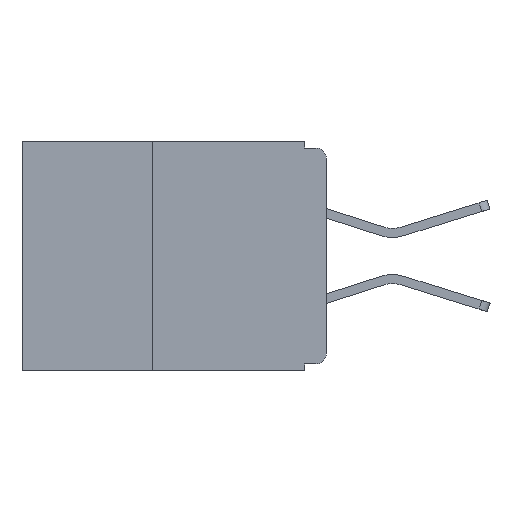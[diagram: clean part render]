
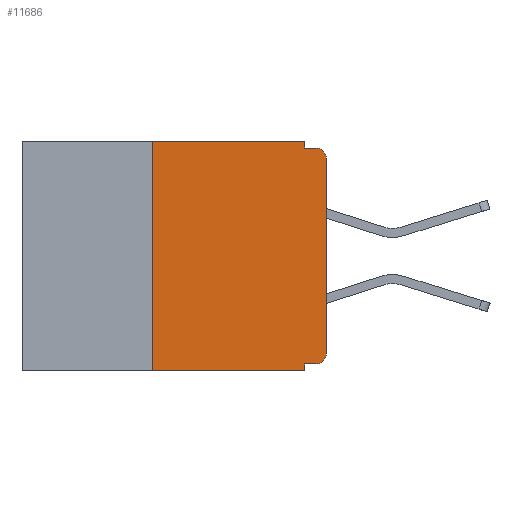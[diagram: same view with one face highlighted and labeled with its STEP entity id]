
A CAD part, left-side view. The second image highlights one B-rep face of the part: STEP entity #11686.
In plain terms, the highlighted planar face has unit normal (-1, 0, 0).
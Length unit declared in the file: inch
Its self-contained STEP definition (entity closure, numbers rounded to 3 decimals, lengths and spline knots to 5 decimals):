
#15 = AXIS2_PLACEMENT_3D ( 'NONE', #8913, #19501, #10410 ) ;
#579 = CARTESIAN_POINT ( 'NONE',  ( 0., 0.015, -0.025 ) ) ;
#1544 = CARTESIAN_POINT ( 'NONE',  ( 0., 0.437, -0.33 ) ) ;
#1584 = LINE ( 'NONE', #1544, #12838 ) ;
#1586 = DIRECTION ( 'NONE',  ( 0., 1., 0. ) ) ;
#1719 = AXIS2_PLACEMENT_3D ( 'NONE', #579, #11249, #2128 ) ;
#2058 = DIRECTION ( 'NONE',  ( 0., -1., 0. ) ) ;
#2121 = CARTESIAN_POINT ( 'NONE',  ( 0., 0., -0.025 ) ) ;
#2128 = DIRECTION ( 'NONE',  ( 0., 0., -1. ) ) ;
#2488 = FACE_OUTER_BOUND ( 'NONE', #13505, .T. ) ;
#2527 = VECTOR ( 'NONE', #3831, 39.37008 ) ;
#3099 = ORIENTED_EDGE ( 'NONE', *, *, #18047, .F. ) ;
#3177 = DIRECTION ( 'NONE',  ( 1., 0., 0. ) ) ;
#3681 = EDGE_CURVE ( 'NONE', #10361, #7495, #19598, .T. ) ;
#3831 = DIRECTION ( 'NONE',  ( 0., 0., -1. ) ) ;
#3846 = CARTESIAN_POINT ( 'NONE',  ( 0., 0.031, -0.33 ) ) ;
#4240 = LINE ( 'NONE', #17031, #7351 ) ;
#4249 = VERTEX_POINT ( 'NONE', #2121 ) ;
#4680 = VERTEX_POINT ( 'NONE', #13640 ) ;
#4694 = CARTESIAN_POINT ( 'NONE',  ( 0., 0., -0.32 ) ) ;
#5428 = EDGE_CURVE ( 'NONE', #9718, #18301, #8872, .T. ) ;
#5846 = EDGE_CURVE ( 'NONE', #14111, #4249, #19669, .T. ) ;
#5915 = VECTOR ( 'NONE', #8288, 39.37008 ) ;
#6095 = VERTEX_POINT ( 'NONE', #7169 ) ;
#6326 = EDGE_CURVE ( 'NONE', #12402, #4680, #18744, .T. ) ;
#7169 = CARTESIAN_POINT ( 'NONE',  ( 0., 0.25, -0.33 ) ) ;
#7178 = ORIENTED_EDGE ( 'NONE', *, *, #5428, .F. ) ;
#7351 = VECTOR ( 'NONE', #7915, 39.37008 ) ;
#7495 = VERTEX_POINT ( 'NONE', #15661 ) ;
#7744 = PLANE ( 'NONE',  #10806 ) ;
#7908 = ORIENTED_EDGE ( 'NONE', *, *, #6326, .F. ) ;
#7915 = DIRECTION ( 'NONE',  ( 0., 0., -1. ) ) ;
#8288 = DIRECTION ( 'NONE',  ( 0., 0., 1. ) ) ;
#8872 = LINE ( 'NONE', #16642, #9338 ) ;
#8913 = CARTESIAN_POINT ( 'NONE',  ( 0., 0.015, -0.305 ) ) ;
#8939 = CARTESIAN_POINT ( 'NONE',  ( 0., 0.25, 0. ) ) ;
#9005 = CARTESIAN_POINT ( 'NONE',  ( 0., 0., -0.01 ) ) ;
#9338 = VECTOR ( 'NONE', #16666, 39.37008 ) ;
#9555 = ORIENTED_EDGE ( 'NONE', *, *, #17956, .T. ) ;
#9718 = VERTEX_POINT ( 'NONE', #8939 ) ;
#10361 = VERTEX_POINT ( 'NONE', #14944 ) ;
#10370 = EDGE_CURVE ( 'NONE', #14925, #14111, #14561, .T. ) ;
#10410 = DIRECTION ( 'NONE',  ( 0., 0., -1. ) ) ;
#10723 = EDGE_CURVE ( 'NONE', #4249, #7495, #15470, .T. ) ;
#10806 = AXIS2_PLACEMENT_3D ( 'NONE', #12309, #3177, #13864 ) ;
#11012 = LINE ( 'NONE', #4694, #14618 ) ;
#11249 = DIRECTION ( 'NONE',  ( -1., 0., 0. ) ) ;
#11269 = EDGE_CURVE ( 'NONE', #6095, #9718, #14053, .T. ) ;
#11291 = CARTESIAN_POINT ( 'NONE',  ( 0., 0., 0. ) ) ;
#11497 = DIRECTION ( 'NONE',  ( 0., 0., 1. ) ) ;
#11686 = ADVANCED_FACE ( 'NONE', ( #2488 ), #7744, .F. ) ;
#11715 = CARTESIAN_POINT ( 'NONE',  ( 0., 0., -0.305 ) ) ;
#12146 = CARTESIAN_POINT ( 'NONE',  ( 0., 0.015, -0.32 ) ) ;
#12309 = CARTESIAN_POINT ( 'NONE',  ( 0., 0.437, 0. ) ) ;
#12402 = VERTEX_POINT ( 'NONE', #19522 ) ;
#12838 = VECTOR ( 'NONE', #15280, 39.37008 ) ;
#13505 = EDGE_LOOP ( 'NONE', ( #15722, #16675, #17652, #3099, #7178, #17187, #9555, #7908, #19747, #16302 ) ) ;
#13640 = CARTESIAN_POINT ( 'NONE',  ( 0., 0.031, -0.33 ) ) ;
#13713 = EDGE_CURVE ( 'NONE', #14925, #12402, #11012, .T. ) ;
#13864 = DIRECTION ( 'NONE',  ( 0., 0., -1. ) ) ;
#14053 = LINE ( 'NONE', #18905, #5915 ) ;
#14111 = VERTEX_POINT ( 'NONE', #11715 ) ;
#14561 = CIRCLE ( 'NONE', #15, 0.015 ) ;
#14618 = VECTOR ( 'NONE', #1586, 39.37008 ) ;
#14925 = VERTEX_POINT ( 'NONE', #12146 ) ;
#14944 = CARTESIAN_POINT ( 'NONE',  ( 0., 0.031, -0.01 ) ) ;
#15280 = DIRECTION ( 'NONE',  ( 0., -1., 0. ) ) ;
#15470 = CIRCLE ( 'NONE', #1719, 0.015 ) ;
#15580 = VECTOR ( 'NONE', #2058, 39.37008 ) ;
#15661 = CARTESIAN_POINT ( 'NONE',  ( 0., 0.015, -0.01 ) ) ;
#15722 = ORIENTED_EDGE ( 'NONE', *, *, #5846, .T. ) ;
#16302 = ORIENTED_EDGE ( 'NONE', *, *, #10370, .T. ) ;
#16642 = CARTESIAN_POINT ( 'NONE',  ( 0., 0.437, 0. ) ) ;
#16666 = DIRECTION ( 'NONE',  ( 0., -1., 0. ) ) ;
#16675 = ORIENTED_EDGE ( 'NONE', *, *, #10723, .T. ) ;
#17031 = CARTESIAN_POINT ( 'NONE',  ( 0., 0.031, 0. ) ) ;
#17187 = ORIENTED_EDGE ( 'NONE', *, *, #11269, .F. ) ;
#17623 = CARTESIAN_POINT ( 'NONE',  ( 0., 0.031, 0. ) ) ;
#17652 = ORIENTED_EDGE ( 'NONE', *, *, #3681, .F. ) ;
#17956 = EDGE_CURVE ( 'NONE', #6095, #4680, #1584, .T. ) ;
#18047 = EDGE_CURVE ( 'NONE', #18301, #10361, #4240, .T. ) ;
#18301 = VERTEX_POINT ( 'NONE', #17623 ) ;
#18744 = LINE ( 'NONE', #3846, #2527 ) ;
#18905 = CARTESIAN_POINT ( 'NONE',  ( 0., 0.25, -0.33 ) ) ;
#19205 = VECTOR ( 'NONE', #11497, 39.37008 ) ;
#19501 = DIRECTION ( 'NONE',  ( -1., 0., 0. ) ) ;
#19522 = CARTESIAN_POINT ( 'NONE',  ( 0., 0.031, -0.32 ) ) ;
#19598 = LINE ( 'NONE', #9005, #15580 ) ;
#19669 = LINE ( 'NONE', #11291, #19205 ) ;
#19747 = ORIENTED_EDGE ( 'NONE', *, *, #13713, .F. ) ;
